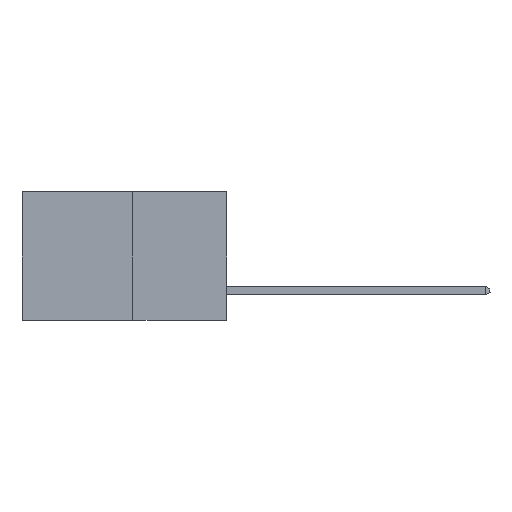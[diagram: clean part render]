
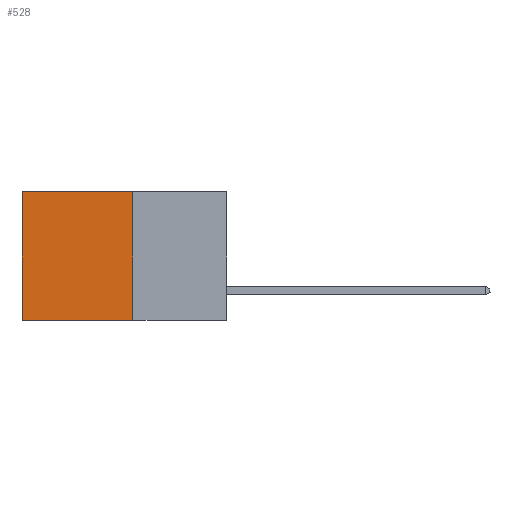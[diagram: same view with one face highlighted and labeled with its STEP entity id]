
A CAD part, left-side view. The second image highlights one B-rep face of the part: STEP entity #528.
In plain terms, the highlighted planar face has unit normal (-1, 0, 0).
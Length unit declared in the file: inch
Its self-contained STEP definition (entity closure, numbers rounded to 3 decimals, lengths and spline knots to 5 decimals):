
#342 = ORIENTED_EDGE ( 'NONE', *, *, #2774, .F. ) ;
#528 = ADVANCED_FACE ( 'NONE', ( #9116 ), #2567, .F. ) ;
#787 = CARTESIAN_POINT ( 'NONE',  ( 0.277, 0.27, -0.37 ) ) ;
#1221 = DIRECTION ( 'NONE',  ( 0., 1., 0. ) ) ;
#1351 = EDGE_CURVE ( 'NONE', #10840, #5115, #8943, .T. ) ;
#1613 = EDGE_LOOP ( 'NONE', ( #12283, #13608, #342, #11062 ) ) ;
#2567 = PLANE ( 'NONE',  #4683 ) ;
#2606 = VERTEX_POINT ( 'NONE', #5944 ) ;
#2774 = EDGE_CURVE ( 'NONE', #2606, #5126, #14835, .T. ) ;
#2959 = CARTESIAN_POINT ( 'NONE',  ( 0.277, 0.59, -0.37 ) ) ;
#3491 = DIRECTION ( 'NONE',  ( 0., 0., -1. ) ) ;
#3537 = DIRECTION ( 'NONE',  ( 1., 0., 0. ) ) ;
#3720 = VECTOR ( 'NONE', #1221, 39.37008 ) ;
#4683 = AXIS2_PLACEMENT_3D ( 'NONE', #787, #3537, #3491 ) ;
#5115 = VERTEX_POINT ( 'NONE', #12360 ) ;
#5126 = VERTEX_POINT ( 'NONE', #14371 ) ;
#5273 = DIRECTION ( 'NONE',  ( 0., 0., -1. ) ) ;
#5593 = CARTESIAN_POINT ( 'NONE',  ( 0.277, 0.27, -0.37 ) ) ;
#5779 = EDGE_CURVE ( 'NONE', #2606, #10840, #12828, .T. ) ;
#5944 = CARTESIAN_POINT ( 'NONE',  ( 0.277, 0.27, 0. ) ) ;
#6032 = VECTOR ( 'NONE', #10097, 39.37008 ) ;
#8566 = VECTOR ( 'NONE', #5273, 39.37008 ) ;
#8831 = CARTESIAN_POINT ( 'NONE',  ( 0.277, 0.27, -0.37 ) ) ;
#8943 = LINE ( 'NONE', #2959, #8566 ) ;
#9116 = FACE_OUTER_BOUND ( 'NONE', #1613, .T. ) ;
#9944 = DIRECTION ( 'NONE',  ( 0., 1., 0. ) ) ;
#10097 = DIRECTION ( 'NONE',  ( 0., 0., -1. ) ) ;
#10313 = EDGE_CURVE ( 'NONE', #5126, #5115, #12559, .T. ) ;
#10840 = VERTEX_POINT ( 'NONE', #10895 ) ;
#10892 = CARTESIAN_POINT ( 'NONE',  ( 0.277, 0.27, 0. ) ) ;
#10895 = CARTESIAN_POINT ( 'NONE',  ( 0.277, 0.59, 0. ) ) ;
#11062 = ORIENTED_EDGE ( 'NONE', *, *, #5779, .T. ) ;
#12283 = ORIENTED_EDGE ( 'NONE', *, *, #1351, .T. ) ;
#12360 = CARTESIAN_POINT ( 'NONE',  ( 0.277, 0.59, -0.37 ) ) ;
#12559 = LINE ( 'NONE', #8831, #14378 ) ;
#12828 = LINE ( 'NONE', #10892, #3720 ) ;
#13608 = ORIENTED_EDGE ( 'NONE', *, *, #10313, .F. ) ;
#14371 = CARTESIAN_POINT ( 'NONE',  ( 0.277, 0.27, -0.37 ) ) ;
#14378 = VECTOR ( 'NONE', #9944, 39.37008 ) ;
#14835 = LINE ( 'NONE', #5593, #6032 ) ;
